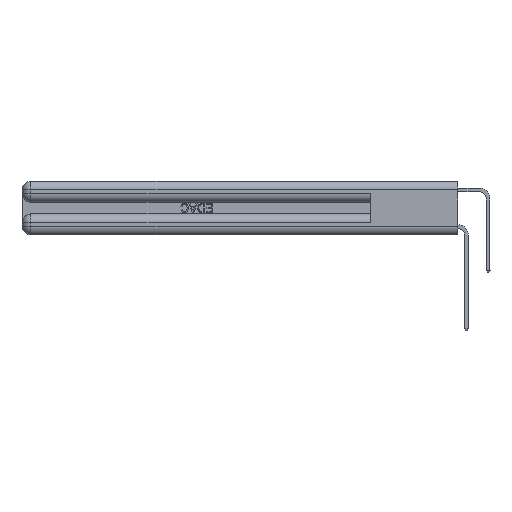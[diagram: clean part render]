
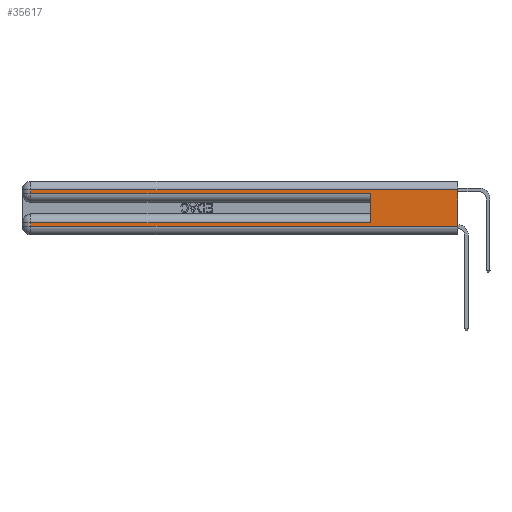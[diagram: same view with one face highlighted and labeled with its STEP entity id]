
A CAD part, left-side view. The second image highlights one B-rep face of the part: STEP entity #35617.
In plain terms, the highlighted planar face has unit normal (-1, 0, 0).
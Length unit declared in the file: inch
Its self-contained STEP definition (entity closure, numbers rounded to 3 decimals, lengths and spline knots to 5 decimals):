
#77 = CARTESIAN_POINT ( 'NONE',  ( 0., 0., 0.37 ) ) ;
#80 = VECTOR ( 'NONE', #27773, 39.37008 ) ;
#132 = VERTEX_POINT ( 'NONE', #30032 ) ;
#400 = LINE ( 'NONE', #28229, #21597 ) ;
#623 = DIRECTION ( 'NONE',  ( 0., -1., 0. ) ) ;
#723 = ORIENTED_EDGE ( 'NONE', *, *, #23173, .T. ) ;
#919 = CARTESIAN_POINT ( 'NONE',  ( 0., 0., 0.285 ) ) ;
#1277 = VERTEX_POINT ( 'NONE', #26005 ) ;
#2003 = LINE ( 'NONE', #4982, #21212 ) ;
#2607 = ORIENTED_EDGE ( 'NONE', *, *, #5724, .T. ) ;
#2671 = EDGE_CURVE ( 'NONE', #30469, #7316, #3580, .T. ) ;
#2810 = DIRECTION ( 'NONE',  ( 0., 0., -1. ) ) ;
#3217 = DIRECTION ( 'NONE',  ( 0., 0., -1. ) ) ;
#3253 = VERTEX_POINT ( 'NONE', #14985 ) ;
#3547 = CARTESIAN_POINT ( 'NONE',  ( 0., 0., 0.31 ) ) ;
#3580 = LINE ( 'NONE', #31398, #12956 ) ;
#4982 = CARTESIAN_POINT ( 'NONE',  ( 0., 0., 0.085 ) ) ;
#5011 = ORIENTED_EDGE ( 'NONE', *, *, #23078, .F. ) ;
#5724 = EDGE_CURVE ( 'NONE', #36071, #3253, #8086, .T. ) ;
#7040 = CARTESIAN_POINT ( 'NONE',  ( 0., 0.6, 0.085 ) ) ;
#7316 = VERTEX_POINT ( 'NONE', #15662 ) ;
#7750 = DIRECTION ( 'NONE',  ( 0., 0., -1. ) ) ;
#8086 = LINE ( 'NONE', #29812, #80 ) ;
#8976 = VERTEX_POINT ( 'NONE', #29324 ) ;
#9263 = CARTESIAN_POINT ( 'NONE',  ( 0., 0.6, 0.145 ) ) ;
#9633 = EDGE_CURVE ( 'NONE', #3253, #8976, #18797, .T. ) ;
#10669 = ORIENTED_EDGE ( 'NONE', *, *, #9633, .T. ) ;
#11750 = FACE_OUTER_BOUND ( 'NONE', #35484, .T. ) ;
#12000 = ORIENTED_EDGE ( 'NONE', *, *, #18135, .F. ) ;
#12088 = CARTESIAN_POINT ( 'NONE',  ( 0., 2.94, 0.06 ) ) ;
#12196 = LINE ( 'NONE', #23395, #13707 ) ;
#12586 = DIRECTION ( 'NONE',  ( 0., -1., 0. ) ) ;
#12956 = VECTOR ( 'NONE', #623, 39.37008 ) ;
#13306 = DIRECTION ( 'NONE',  ( 0., 1., 0. ) ) ;
#13422 = VECTOR ( 'NONE', #20127, 39.37008 ) ;
#13707 = VECTOR ( 'NONE', #31852, 39.37008 ) ;
#14232 = VERTEX_POINT ( 'NONE', #7040 ) ;
#14985 = CARTESIAN_POINT ( 'NONE',  ( 0., 2.94, 0.31 ) ) ;
#15662 = CARTESIAN_POINT ( 'NONE',  ( 0., 0., 0.06 ) ) ;
#18135 = EDGE_CURVE ( 'NONE', #36071, #7316, #400, .T. ) ;
#18797 = LINE ( 'NONE', #36085, #28561 ) ;
#19204 = ORIENTED_EDGE ( 'NONE', *, *, #33564, .T. ) ;
#19934 = ORIENTED_EDGE ( 'NONE', *, *, #29353, .T. ) ;
#20127 = DIRECTION ( 'NONE',  ( 0., 0., 1. ) ) ;
#21212 = VECTOR ( 'NONE', #13306, 39.37008 ) ;
#21597 = VECTOR ( 'NONE', #2810, 39.37008 ) ;
#22002 = AXIS2_PLACEMENT_3D ( 'NONE', #77, #28442, #3217 ) ;
#23078 = EDGE_CURVE ( 'NONE', #14232, #1277, #28376, .T. ) ;
#23173 = EDGE_CURVE ( 'NONE', #8976, #1277, #28929, .T. ) ;
#23395 = CARTESIAN_POINT ( 'NONE',  ( 0., 2.94, 0.37 ) ) ;
#24484 = ORIENTED_EDGE ( 'NONE', *, *, #2671, .T. ) ;
#26005 = CARTESIAN_POINT ( 'NONE',  ( 0., 0.6, 0.285 ) ) ;
#26295 = VECTOR ( 'NONE', #12586, 39.37008 ) ;
#27773 = DIRECTION ( 'NONE',  ( 0., 1., 0. ) ) ;
#28229 = CARTESIAN_POINT ( 'NONE',  ( 0., 0., 0.37 ) ) ;
#28376 = LINE ( 'NONE', #9263, #13422 ) ;
#28442 = DIRECTION ( 'NONE',  ( 1., 0., 0. ) ) ;
#28561 = VECTOR ( 'NONE', #7750, 39.37008 ) ;
#28929 = LINE ( 'NONE', #919, #26295 ) ;
#29324 = CARTESIAN_POINT ( 'NONE',  ( 0., 2.94, 0.285 ) ) ;
#29353 = EDGE_CURVE ( 'NONE', #14232, #132, #2003, .T. ) ;
#29812 = CARTESIAN_POINT ( 'NONE',  ( 0., 0., 0.31 ) ) ;
#30032 = CARTESIAN_POINT ( 'NONE',  ( 0., 2.94, 0.085 ) ) ;
#30469 = VERTEX_POINT ( 'NONE', #12088 ) ;
#31398 = CARTESIAN_POINT ( 'NONE',  ( 0., 0., 0.06 ) ) ;
#31852 = DIRECTION ( 'NONE',  ( 0., 0., -1. ) ) ;
#33564 = EDGE_CURVE ( 'NONE', #132, #30469, #12196, .T. ) ;
#33805 = PLANE ( 'NONE',  #22002 ) ;
#35484 = EDGE_LOOP ( 'NONE', ( #12000, #2607, #10669, #723, #5011, #19934, #19204, #24484 ) ) ;
#35617 = ADVANCED_FACE ( 'NONE', ( #11750 ), #33805, .F. ) ;
#36071 = VERTEX_POINT ( 'NONE', #3547 ) ;
#36085 = CARTESIAN_POINT ( 'NONE',  ( 0., 2.94, 0.37 ) ) ;
